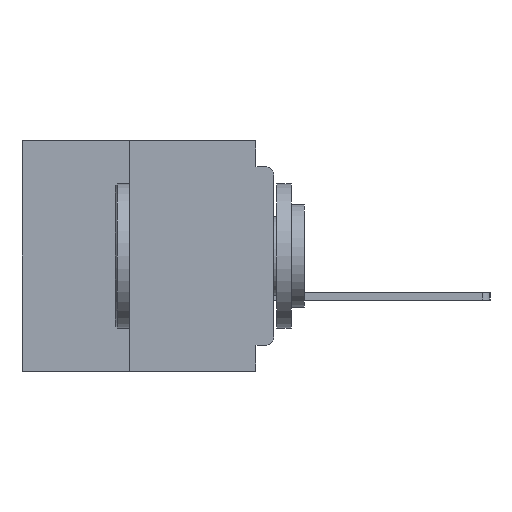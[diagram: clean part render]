
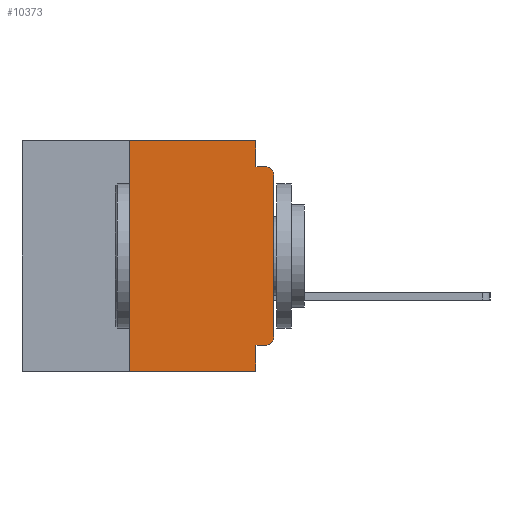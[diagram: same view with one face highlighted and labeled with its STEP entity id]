
A CAD part, left-side view. The second image highlights one B-rep face of the part: STEP entity #10373.
In plain terms, the highlighted planar face has unit normal (-1, 0, 0).
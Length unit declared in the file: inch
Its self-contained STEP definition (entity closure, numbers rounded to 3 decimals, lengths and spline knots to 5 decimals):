
#119 = DIRECTION ( 'NONE',  ( 0., 1., 0. ) ) ;
#214 = ORIENTED_EDGE ( 'NONE', *, *, #16570, .F. ) ;
#357 = ORIENTED_EDGE ( 'NONE', *, *, #38501, .T. ) ;
#515 = ORIENTED_EDGE ( 'NONE', *, *, #2372, .T. ) ;
#600 = LINE ( 'NONE', #36272, #10006 ) ;
#1552 = AXIS2_PLACEMENT_3D ( 'NONE', #27462, #6405, #31005 ) ;
#1651 = VECTOR ( 'NONE', #119, 39.37008 ) ;
#1725 = VERTEX_POINT ( 'NONE', #12336 ) ;
#2019 = VERTEX_POINT ( 'NONE', #23388 ) ;
#2023 = DIRECTION ( 'NONE',  ( 0., 0., -1. ) ) ;
#2372 = EDGE_CURVE ( 'NONE', #16321, #25596, #11517, .T. ) ;
#2779 = DIRECTION ( 'NONE',  ( 0., -1., 0. ) ) ;
#2843 = LINE ( 'NONE', #30643, #20478 ) ;
#2927 = ORIENTED_EDGE ( 'NONE', *, *, #14754, .F. ) ;
#3637 = CARTESIAN_POINT ( 'NONE',  ( 0., 0., -0.34 ) ) ;
#4039 = LINE ( 'NONE', #42677, #23827 ) ;
#4112 = VERTEX_POINT ( 'NONE', #15860 ) ;
#4826 = EDGE_LOOP ( 'NONE', ( #28519, #515, #6027, #11024, #30998, #31619, #32167, #2927, #214, #357 ) ) ;
#5380 = DIRECTION ( 'NONE',  ( 0., 0., -1. ) ) ;
#6027 = ORIENTED_EDGE ( 'NONE', *, *, #35339, .F. ) ;
#6405 = DIRECTION ( 'NONE',  ( -1., 0., 0. ) ) ;
#6826 = EDGE_CURVE ( 'NONE', #32846, #21073, #600, .T. ) ;
#8274 = AXIS2_PLACEMENT_3D ( 'NONE', #32416, #32331, #31874 ) ;
#9066 = VECTOR ( 'NONE', #2023, 39.37008 ) ;
#9329 = CARTESIAN_POINT ( 'NONE',  ( 0., 0.25, -0.4 ) ) ;
#9735 = CARTESIAN_POINT ( 'NONE',  ( 0., 0.437, -0.4 ) ) ;
#10006 = VECTOR ( 'NONE', #25547, 39.37008 ) ;
#10373 = ADVANCED_FACE ( 'NONE', ( #29410 ), #15922, .F. ) ;
#10685 = VECTOR ( 'NONE', #30368, 39.37008 ) ;
#11024 = ORIENTED_EDGE ( 'NONE', *, *, #35848, .F. ) ;
#11251 = DIRECTION ( 'NONE',  ( 0., 0., -1. ) ) ;
#11517 = CIRCLE ( 'NONE', #8274, 0.015 ) ;
#12336 = CARTESIAN_POINT ( 'NONE',  ( 0., 0.25, -0.4 ) ) ;
#12724 = VERTEX_POINT ( 'NONE', #3637 ) ;
#12945 = CARTESIAN_POINT ( 'NONE',  ( 0., 0., -0.06 ) ) ;
#13062 = CARTESIAN_POINT ( 'NONE',  ( 0., 0.031, -0.355 ) ) ;
#13566 = VECTOR ( 'NONE', #41274, 39.37008 ) ;
#14754 = EDGE_CURVE ( 'NONE', #20598, #4112, #4039, .T. ) ;
#15707 = EDGE_CURVE ( 'NONE', #12724, #16321, #2843, .T. ) ;
#15860 = CARTESIAN_POINT ( 'NONE',  ( 0., 0.031, -0.4 ) ) ;
#15922 = PLANE ( 'NONE',  #24427 ) ;
#16321 = VERTEX_POINT ( 'NONE', #12945 ) ;
#16570 = EDGE_CURVE ( 'NONE', #42052, #20598, #19299, .T. ) ;
#18460 = LINE ( 'NONE', #23064, #9066 ) ;
#19299 = LINE ( 'NONE', #24708, #1651 ) ;
#19335 = CARTESIAN_POINT ( 'NONE',  ( 0., 0.015, -0.045 ) ) ;
#19420 = CARTESIAN_POINT ( 'NONE',  ( 0., 0.437, 0. ) ) ;
#19473 = CARTESIAN_POINT ( 'NONE',  ( 0., 0.031, 0. ) ) ;
#20395 = CARTESIAN_POINT ( 'NONE',  ( 0., 0., -0.045 ) ) ;
#20478 = VECTOR ( 'NONE', #40955, 39.37008 ) ;
#20598 = VERTEX_POINT ( 'NONE', #13062 ) ;
#21073 = VERTEX_POINT ( 'NONE', #19473 ) ;
#21765 = EDGE_CURVE ( 'NONE', #1725, #4112, #26612, .T. ) ;
#23064 = CARTESIAN_POINT ( 'NONE',  ( 0., 0.031, 0. ) ) ;
#23388 = CARTESIAN_POINT ( 'NONE',  ( 0., 0.031, -0.045 ) ) ;
#23827 = VECTOR ( 'NONE', #11251, 39.37008 ) ;
#24427 = AXIS2_PLACEMENT_3D ( 'NONE', #19420, #26425, #5380 ) ;
#24708 = CARTESIAN_POINT ( 'NONE',  ( 0., 0., -0.355 ) ) ;
#25547 = DIRECTION ( 'NONE',  ( 0., -1., 0. ) ) ;
#25596 = VERTEX_POINT ( 'NONE', #19335 ) ;
#26418 = CARTESIAN_POINT ( 'NONE',  ( 0., 0.25, 0. ) ) ;
#26425 = DIRECTION ( 'NONE',  ( 1., 0., 0. ) ) ;
#26612 = LINE ( 'NONE', #9735, #43968 ) ;
#27462 = CARTESIAN_POINT ( 'NONE',  ( 0., 0.015, -0.34 ) ) ;
#28519 = ORIENTED_EDGE ( 'NONE', *, *, #15707, .T. ) ;
#28814 = EDGE_CURVE ( 'NONE', #1725, #32846, #44486, .T. ) ;
#29410 = FACE_OUTER_BOUND ( 'NONE', #4826, .T. ) ;
#30368 = DIRECTION ( 'NONE',  ( 0., 0., 1. ) ) ;
#30643 = CARTESIAN_POINT ( 'NONE',  ( 0., 0., 0. ) ) ;
#30998 = ORIENTED_EDGE ( 'NONE', *, *, #6826, .F. ) ;
#31005 = DIRECTION ( 'NONE',  ( 0., 0., -1. ) ) ;
#31619 = ORIENTED_EDGE ( 'NONE', *, *, #28814, .F. ) ;
#31874 = DIRECTION ( 'NONE',  ( 0., 0., -1. ) ) ;
#32167 = ORIENTED_EDGE ( 'NONE', *, *, #21765, .T. ) ;
#32331 = DIRECTION ( 'NONE',  ( -1., 0., 0. ) ) ;
#32416 = CARTESIAN_POINT ( 'NONE',  ( 0., 0.015, -0.06 ) ) ;
#32846 = VERTEX_POINT ( 'NONE', #26418 ) ;
#34854 = CIRCLE ( 'NONE', #1552, 0.015 ) ;
#35339 = EDGE_CURVE ( 'NONE', #2019, #25596, #41420, .T. ) ;
#35708 = CARTESIAN_POINT ( 'NONE',  ( 0., 0.015, -0.355 ) ) ;
#35848 = EDGE_CURVE ( 'NONE', #21073, #2019, #18460, .T. ) ;
#36272 = CARTESIAN_POINT ( 'NONE',  ( 0., 0.437, 0. ) ) ;
#38501 = EDGE_CURVE ( 'NONE', #42052, #12724, #34854, .T. ) ;
#40955 = DIRECTION ( 'NONE',  ( 0., 0., 1. ) ) ;
#41274 = DIRECTION ( 'NONE',  ( 0., -1., 0. ) ) ;
#41420 = LINE ( 'NONE', #20395, #13566 ) ;
#42052 = VERTEX_POINT ( 'NONE', #35708 ) ;
#42677 = CARTESIAN_POINT ( 'NONE',  ( 0., 0.031, -0.4 ) ) ;
#43968 = VECTOR ( 'NONE', #2779, 39.37008 ) ;
#44486 = LINE ( 'NONE', #9329, #10685 ) ;
